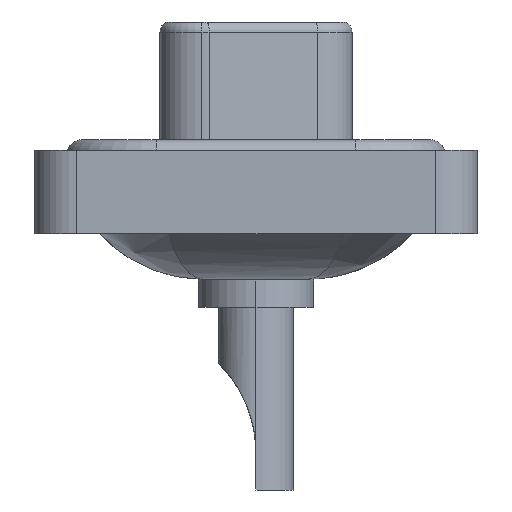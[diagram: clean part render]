
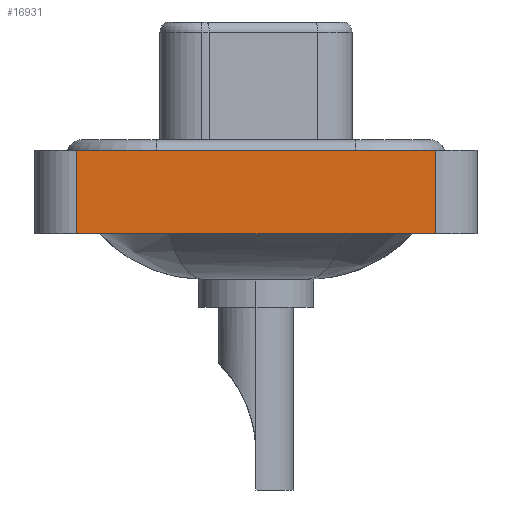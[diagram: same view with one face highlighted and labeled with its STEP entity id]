
A CAD part, left-side view. The second image highlights one B-rep face of the part: STEP entity #16931.
In plain terms, the highlighted planar face has unit normal (-1, 0, 0).
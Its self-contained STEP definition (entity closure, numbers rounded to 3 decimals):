
#968 = VERTEX_POINT ( 'NONE', #6157 ) ;
#1969 = EDGE_CURVE ( 'NONE', #16570, #968, #16076, .T. ) ;
#2151 = VECTOR ( 'NONE', #12492, 1000. ) ;
#2548 = FACE_OUTER_BOUND ( 'NONE', #7144, .T. ) ;
#2757 = CARTESIAN_POINT ( 'NONE',  ( -7.3, 8.55, -3.6 ) ) ;
#3947 = DIRECTION ( 'NONE',  ( 0., 0., 1. ) ) ;
#3982 = EDGE_CURVE ( 'NONE', #15920, #16570, #19646, .T. ) ;
#4239 = VECTOR ( 'NONE', #19176, 1000. ) ;
#4392 = EDGE_CURVE ( 'NONE', #4936, #968, #11909, .T. ) ;
#4776 = VECTOR ( 'NONE', #8900, 1000. ) ;
#4817 = CARTESIAN_POINT ( 'NONE',  ( -7.3, 8.55, -3.6 ) ) ;
#4936 = VERTEX_POINT ( 'NONE', #16800 ) ;
#5604 = EDGE_CURVE ( 'NONE', #15920, #4936, #11194, .T. ) ;
#5654 = DIRECTION ( 'NONE',  ( -1., 0., 0. ) ) ;
#5701 = ORIENTED_EDGE ( 'NONE', *, *, #3982, .F. ) ;
#6157 = CARTESIAN_POINT ( 'NONE',  ( -7.3, -8.55, 0.4 ) ) ;
#7144 = EDGE_LOOP ( 'NONE', ( #16619, #12876, #5701, #18829 ) ) ;
#8044 = CARTESIAN_POINT ( 'NONE',  ( -7.3, -8.55, -3.6 ) ) ;
#8900 = DIRECTION ( 'NONE',  ( 0., 0., 1. ) ) ;
#10148 = CARTESIAN_POINT ( 'NONE',  ( -7.3, -8.55, 0.4 ) ) ;
#11194 = LINE ( 'NONE', #8044, #2151 ) ;
#11909 = LINE ( 'NONE', #16540, #13819 ) ;
#12492 = DIRECTION ( 'NONE',  ( 0., -1., 0. ) ) ;
#12876 = ORIENTED_EDGE ( 'NONE', *, *, #1969, .F. ) ;
#13032 = DIRECTION ( 'NONE',  ( 0., 0., 1. ) ) ;
#13819 = VECTOR ( 'NONE', #3947, 1000. ) ;
#15920 = VERTEX_POINT ( 'NONE', #4817 ) ;
#16076 = LINE ( 'NONE', #10148, #4239 ) ;
#16540 = CARTESIAN_POINT ( 'NONE',  ( -7.3, -8.55, -3.6 ) ) ;
#16570 = VERTEX_POINT ( 'NONE', #19364 ) ;
#16619 = ORIENTED_EDGE ( 'NONE', *, *, #4392, .T. ) ;
#16800 = CARTESIAN_POINT ( 'NONE',  ( -7.3, -8.55, -3.6 ) ) ;
#16931 = ADVANCED_FACE ( 'NONE', ( #2548 ), #17959, .T. ) ;
#17959 = PLANE ( 'NONE',  #19137 ) ;
#18829 = ORIENTED_EDGE ( 'NONE', *, *, #5604, .T. ) ;
#19137 = AXIS2_PLACEMENT_3D ( 'NONE', #19242, #5654, #13032 ) ;
#19176 = DIRECTION ( 'NONE',  ( 0., -1., 0. ) ) ;
#19242 = CARTESIAN_POINT ( 'NONE',  ( -7.3, -8.55, -3.6 ) ) ;
#19364 = CARTESIAN_POINT ( 'NONE',  ( -7.3, 8.55, 0.4 ) ) ;
#19646 = LINE ( 'NONE', #2757, #4776 ) ;
